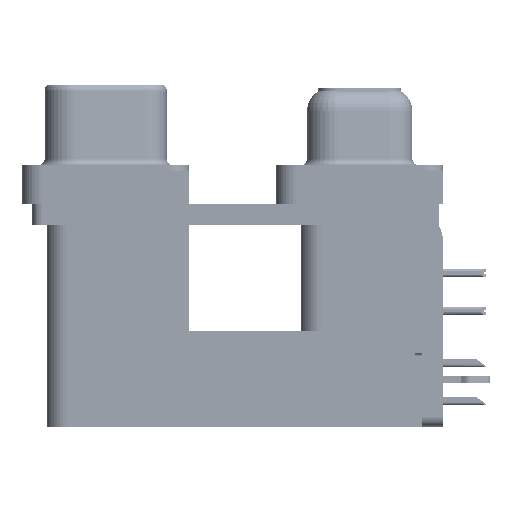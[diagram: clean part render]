
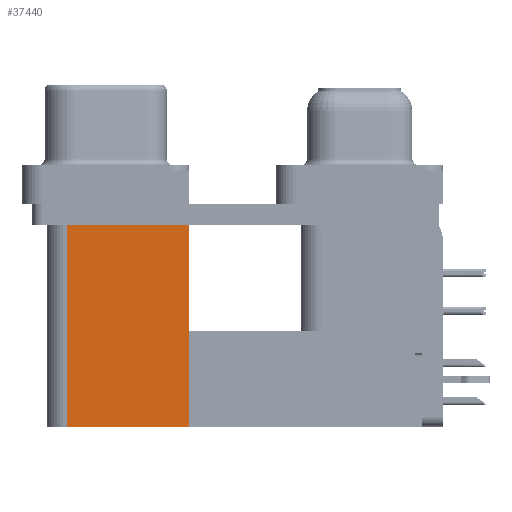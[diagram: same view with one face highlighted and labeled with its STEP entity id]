
A CAD part, left-side view. The second image highlights one B-rep face of the part: STEP entity #37440.
In plain terms, the highlighted planar face has unit normal (-1, 0, 0).
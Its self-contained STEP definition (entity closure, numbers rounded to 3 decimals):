
#1330 = VERTEX_POINT ( 'NONE', #20198 ) ;
#1584 = EDGE_CURVE ( 'NONE', #2453, #1330, #64465, .T. ) ;
#2453 = VERTEX_POINT ( 'NONE', #9820 ) ;
#5932 = FACE_OUTER_BOUND ( 'NONE', #50249, .T. ) ;
#5994 = LINE ( 'NONE', #63133, #68116 ) ;
#6989 = DIRECTION ( 'NONE',  ( 1., 0., 0. ) ) ;
#9820 = CARTESIAN_POINT ( 'NONE',  ( 3.79, 12.775, -19.2 ) ) ;
#13644 = ORIENTED_EDGE ( 'NONE', *, *, #39712, .F. ) ;
#14927 = DIRECTION ( 'NONE',  ( 0., 0., 1. ) ) ;
#14955 = LINE ( 'NONE', #41752, #30247 ) ;
#15691 = VERTEX_POINT ( 'NONE', #41861 ) ;
#20198 = CARTESIAN_POINT ( 'NONE',  ( 3.79, 21.975, -19.2 ) ) ;
#23185 = CARTESIAN_POINT ( 'NONE',  ( 3.79, 12.775, -19.2 ) ) ;
#26591 = CARTESIAN_POINT ( 'NONE',  ( 3.79, 21.975, -19.2 ) ) ;
#27237 = VECTOR ( 'NONE', #50781, 1000. ) ;
#28270 = CARTESIAN_POINT ( 'NONE',  ( 3.79, 12.775, -19.2 ) ) ;
#28864 = ORIENTED_EDGE ( 'NONE', *, *, #66433, .T. ) ;
#29157 = VECTOR ( 'NONE', #47715, 1000. ) ;
#29212 = ORIENTED_EDGE ( 'NONE', *, *, #1584, .F. ) ;
#30247 = VECTOR ( 'NONE', #30841, 1000. ) ;
#30841 = DIRECTION ( 'NONE',  ( 0., 1., 0. ) ) ;
#32222 = LINE ( 'NONE', #26591, #29157 ) ;
#34086 = EDGE_CURVE ( 'NONE', #2453, #53417, #5994, .T. ) ;
#37440 = ADVANCED_FACE ( 'NONE', ( #5932 ), #48905, .F. ) ;
#39712 = EDGE_CURVE ( 'NONE', #1330, #15691, #32222, .T. ) ;
#41752 = CARTESIAN_POINT ( 'NONE',  ( 3.79, 12.775, -2.5 ) ) ;
#41861 = CARTESIAN_POINT ( 'NONE',  ( 3.79, 21.975, -2.5 ) ) ;
#47715 = DIRECTION ( 'NONE',  ( 0., 0., 1. ) ) ;
#48905 = PLANE ( 'NONE',  #57087 ) ;
#50249 = EDGE_LOOP ( 'NONE', ( #28864, #13644, #29212, #50940 ) ) ;
#50781 = DIRECTION ( 'NONE',  ( 0., 1., 0. ) ) ;
#50940 = ORIENTED_EDGE ( 'NONE', *, *, #34086, .T. ) ;
#53249 = CARTESIAN_POINT ( 'NONE',  ( 3.79, 12.775, -2.5 ) ) ;
#53417 = VERTEX_POINT ( 'NONE', #53249 ) ;
#57087 = AXIS2_PLACEMENT_3D ( 'NONE', #23185, #6989, #66097 ) ;
#63133 = CARTESIAN_POINT ( 'NONE',  ( 3.79, 12.775, -19.2 ) ) ;
#64465 = LINE ( 'NONE', #28270, #27237 ) ;
#66097 = DIRECTION ( 'NONE',  ( 0., 1., 0. ) ) ;
#66433 = EDGE_CURVE ( 'NONE', #53417, #15691, #14955, .T. ) ;
#68116 = VECTOR ( 'NONE', #14927, 1000. ) ;
